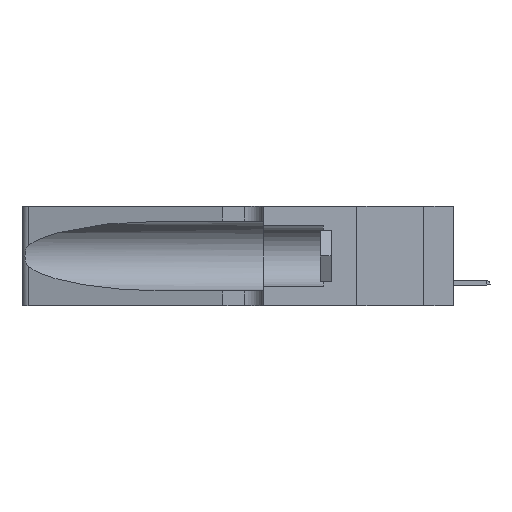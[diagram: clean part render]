
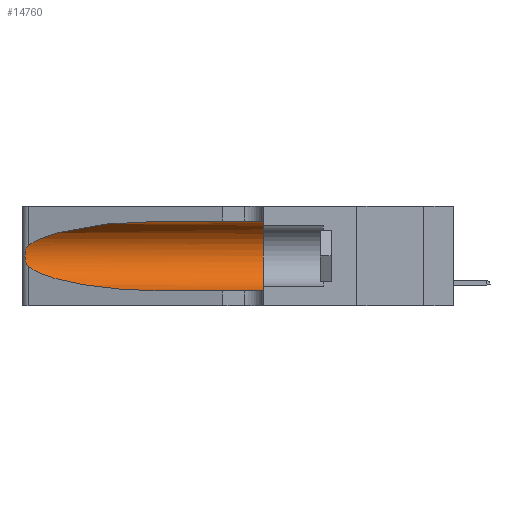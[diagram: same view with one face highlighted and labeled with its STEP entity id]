
A CAD part, left-side view. The second image highlights one B-rep face of the part: STEP entity #14760.
In plain terms, the highlighted cylindrical face has radius 3.308 mm (diameter 6.617 mm), a partial arc.
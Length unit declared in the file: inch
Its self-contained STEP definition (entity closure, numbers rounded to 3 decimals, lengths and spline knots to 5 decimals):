
#422 = CARTESIAN_POINT ( 'NONE',  ( 0.1305, 1.61858, 0.31525 ) ) ;
#837 = VERTEX_POINT ( 'NONE', #49233 ) ;
#1173 = CARTESIAN_POINT ( 'NONE',  ( 0.26018, 1.23835, 0.19895 ) ) ;
#4051 = EDGE_CURVE ( 'NONE', #22204, #24084, #28138, .T. ) ;
#5483 = VERTEX_POINT ( 'NONE', #39485 ) ;
#5880 = EDGE_LOOP ( 'NONE', ( #35682, #44829, #24360, #6928, #27816, #29724 ) ) ;
#6247 = CARTESIAN_POINT ( 'NONE',  ( 0.25487, 1.22718, 0.22369 ) ) ;
#6928 = ORIENTED_EDGE ( 'NONE', *, *, #4051, .T. ) ;
#9637 = CARTESIAN_POINT ( 'NONE',  ( 0.25555, 1.22994, 0.2215 ) ) ;
#9890 = CARTESIAN_POINT ( 'NONE',  ( 0.25555, 1.22993, 0.14849 ) ) ;
#10358 = CARTESIAN_POINT ( 'NONE',  ( 0.2373, 1.15595, 0.28018 ) ) ;
#10551 = VECTOR ( 'NONE', #47340, 39.37008 ) ;
#11142 = CARTESIAN_POINT ( 'NONE',  ( 0.1305, 1.61858, 0.185 ) ) ;
#12090 = CARTESIAN_POINT ( 'NONE',  ( 0.1305, 0.72297, 0.05475 ) ) ;
#12148 = CARTESIAN_POINT ( 'NONE',  ( 0.1305, 0.72297, 0.05475 ) ) ;
#13692 = CARTESIAN_POINT ( 'NONE',  ( 0.18966, 0.96281, 0.31525 ) ) ;
#14760 = ADVANCED_FACE ( 'NONE', ( #38317 ), #33719, .F. ) ;
#14895 = VERTEX_POINT ( 'NONE', #43664 ) ;
#16068 = DIRECTION ( 'NONE',  ( 0., -1., 0. ) ) ;
#17603 = AXIS2_PLACEMENT_3D ( 'NONE', #11142, #41909, #45764 ) ;
#18083 = CARTESIAN_POINT ( 'NONE',  ( 0.26075, 1.23896, 0.178 ) ) ;
#20668 = CARTESIAN_POINT ( 'NONE',  ( 0.25854, 1.2359, 0.20912 ) ) ;
#20749 =( BOUNDED_CURVE ( )  B_SPLINE_CURVE ( 3, ( #33446, #13692, #10358, #6247 ),
 .UNSPECIFIED., .F., .T. ) 
 B_SPLINE_CURVE_WITH_KNOTS ( ( 4, 4 ),
 ( 1.5708, 2.84003 ),
 .UNSPECIFIED. ) 
 CURVE ( )  GEOMETRIC_REPRESENTATION_ITEM ( )  RATIONAL_B_SPLINE_CURVE ( ( 1., 0.87, 0.87, 1. ) ) 
 REPRESENTATION_ITEM ( '' )  );
#21423 = CARTESIAN_POINT ( 'NONE',  ( 0.26017, 1.23833, 0.17102 ) ) ;
#22204 = VERTEX_POINT ( 'NONE', #12090 ) ;
#23145 = VERTEX_POINT ( 'NONE', #41620 ) ;
#23444 = CARTESIAN_POINT ( 'NONE',  ( 0.25487, 1.22718, 0.14631 ) ) ;
#24084 = VERTEX_POINT ( 'NONE', #39737 ) ;
#24360 = ORIENTED_EDGE ( 'NONE', *, *, #26530, .T. ) ;
#25079 = CARTESIAN_POINT ( 'NONE',  ( 0.1305, 0.35, 0.185 ) ) ;
#26530 = EDGE_CURVE ( 'NONE', #23145, #22204, #27652, .T. ) ;
#27549 = CARTESIAN_POINT ( 'NONE',  ( 0.18966, 0.96281, 0.05475 ) ) ;
#27652 =( BOUNDED_CURVE ( )  B_SPLINE_CURVE ( 3, ( #23444, #42682, #27549, #12148 ),
 .UNSPECIFIED., .F., .F. ) 
 B_SPLINE_CURVE_WITH_KNOTS ( ( 4, 4 ),
 ( 3.44316, 4.71239 ),
 .UNSPECIFIED. ) 
 CURVE ( )  GEOMETRIC_REPRESENTATION_ITEM ( )  RATIONAL_B_SPLINE_CURVE ( ( 1., 0.87, 0.87, 1. ) ) 
 REPRESENTATION_ITEM ( '' )  );
#27816 = ORIENTED_EDGE ( 'NONE', *, *, #44006, .F. ) ;
#27867 = LINE ( 'NONE', #422, #10551 ) ;
#28138 = LINE ( 'NONE', #39167, #45972 ) ;
#29724 = ORIENTED_EDGE ( 'NONE', *, *, #30955, .F. ) ;
#30155 = CARTESIAN_POINT ( 'NONE',  ( 0.25856, 1.23593, 0.16098 ) ) ;
#30955 = EDGE_CURVE ( 'NONE', #14895, #837, #27867, .T. ) ;
#31726 = B_SPLINE_CURVE_WITH_KNOTS ( 'NONE', 3,
 ( #32973, #9637, #47839, #43999, #20668, #1173, #45524, #18083, #21423, #30155, #41929, #37324, #9890, #40917 ),
 .UNSPECIFIED., .F., .F.,
 ( 4, 2, 2, 2, 2, 2, 4 ),
 ( 0., 0.00027, 0.00053, 0.00107, 0.0016, 0.00187, 0.00214 ),
 .UNSPECIFIED. ) ;
#32973 = CARTESIAN_POINT ( 'NONE',  ( 0.25487, 1.22718, 0.22369 ) ) ;
#33446 = CARTESIAN_POINT ( 'NONE',  ( 0.1305, 0.72297, 0.31525 ) ) ;
#33719 = CYLINDRICAL_SURFACE ( 'NONE', #17603, 0.13025 ) ;
#35682 = ORIENTED_EDGE ( 'NONE', *, *, #48537, .T. ) ;
#35784 = EDGE_CURVE ( 'NONE', #5483, #23145, #31726, .T. ) ;
#37324 = CARTESIAN_POINT ( 'NONE',  ( 0.25639, 1.23186, 0.15144 ) ) ;
#37376 = DIRECTION ( 'NONE',  ( 0., 0., 1. ) ) ;
#37533 = AXIS2_PLACEMENT_3D ( 'NONE', #25079, #40718, #37376 ) ;
#38317 = FACE_OUTER_BOUND ( 'NONE', #5880, .T. ) ;
#39145 = CIRCLE ( 'NONE', #37533, 0.13025 ) ;
#39167 = CARTESIAN_POINT ( 'NONE',  ( 0.1305, 1.61858, 0.05475 ) ) ;
#39485 = CARTESIAN_POINT ( 'NONE',  ( 0.25487, 1.22718, 0.22369 ) ) ;
#39737 = CARTESIAN_POINT ( 'NONE',  ( 0.1305, 0.35, 0.05475 ) ) ;
#40718 = DIRECTION ( 'NONE',  ( 0., 1., 0. ) ) ;
#40917 = CARTESIAN_POINT ( 'NONE',  ( 0.25487, 1.22718, 0.14631 ) ) ;
#41620 = CARTESIAN_POINT ( 'NONE',  ( 0.25487, 1.22718, 0.14631 ) ) ;
#41909 = DIRECTION ( 'NONE',  ( 0., -1., 0. ) ) ;
#41929 = CARTESIAN_POINT ( 'NONE',  ( 0.25789, 1.23486, 0.15765 ) ) ;
#42682 = CARTESIAN_POINT ( 'NONE',  ( 0.2373, 1.15595, 0.08982 ) ) ;
#43664 = CARTESIAN_POINT ( 'NONE',  ( 0.1305, 0.72297, 0.31525 ) ) ;
#43999 = CARTESIAN_POINT ( 'NONE',  ( 0.25787, 1.23484, 0.2124 ) ) ;
#44006 = EDGE_CURVE ( 'NONE', #837, #24084, #39145, .T. ) ;
#44829 = ORIENTED_EDGE ( 'NONE', *, *, #35784, .T. ) ;
#45524 = CARTESIAN_POINT ( 'NONE',  ( 0.26075, 1.23896, 0.19203 ) ) ;
#45764 = DIRECTION ( 'NONE',  ( 0., 0., -1. ) ) ;
#45972 = VECTOR ( 'NONE', #16068, 39.37008 ) ;
#47340 = DIRECTION ( 'NONE',  ( 0., -1., 0. ) ) ;
#47839 = CARTESIAN_POINT ( 'NONE',  ( 0.25639, 1.23184, 0.21858 ) ) ;
#48537 = EDGE_CURVE ( 'NONE', #14895, #5483, #20749, .T. ) ;
#49233 = CARTESIAN_POINT ( 'NONE',  ( 0.1305, 0.35, 0.31525 ) ) ;
